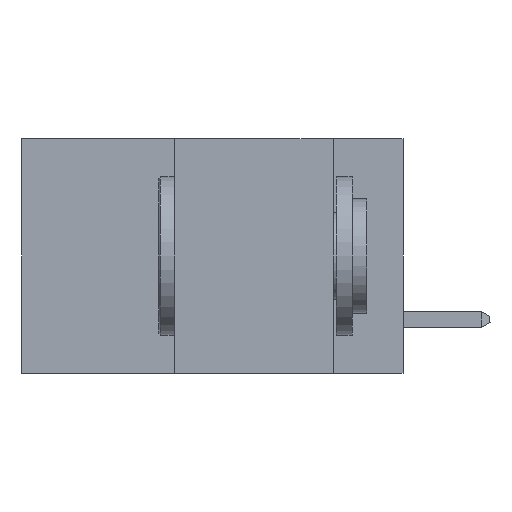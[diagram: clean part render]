
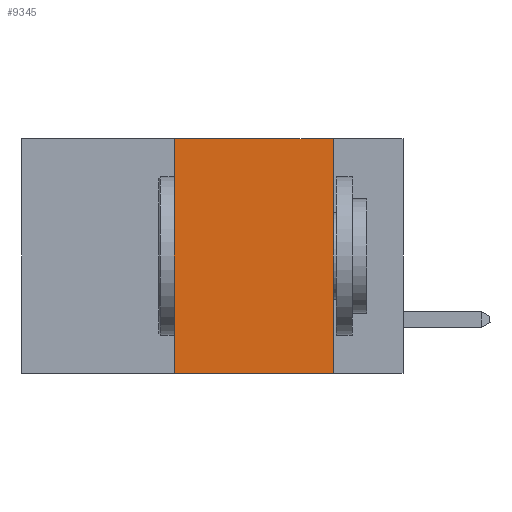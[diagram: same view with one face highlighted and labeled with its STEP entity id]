
A CAD part, left-side view. The second image highlights one B-rep face of the part: STEP entity #9345.
In plain terms, the highlighted planar face has unit normal (-1, 0, 0).
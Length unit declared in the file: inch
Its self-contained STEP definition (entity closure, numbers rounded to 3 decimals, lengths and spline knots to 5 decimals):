
#1799 = CARTESIAN_POINT ( 'NONE',  ( 0., 0.11, -0.37 ) ) ;
#2790 = ORIENTED_EDGE ( 'NONE', *, *, #40341, .F. ) ;
#2924 = ORIENTED_EDGE ( 'NONE', *, *, #37713, .T. ) ;
#2994 = FACE_OUTER_BOUND ( 'NONE', #41935, .T. ) ;
#3256 = LINE ( 'NONE', #39572, #8671 ) ;
#4852 = DIRECTION ( 'NONE',  ( 0., 0., 1. ) ) ;
#5921 = VECTOR ( 'NONE', #29183, 39.37008 ) ;
#8671 = VECTOR ( 'NONE', #4852, 39.37008 ) ;
#9345 = ADVANCED_FACE ( 'NONE', ( #2994 ), #28488, .F. ) ;
#12710 = ORIENTED_EDGE ( 'NONE', *, *, #32119, .F. ) ;
#13232 = VECTOR ( 'NONE', #44209, 39.37008 ) ;
#13265 = CARTESIAN_POINT ( 'NONE',  ( 0., 0.36, -0.37 ) ) ;
#17133 = CARTESIAN_POINT ( 'NONE',  ( 0., 0.6, -0.37 ) ) ;
#17920 = EDGE_CURVE ( 'NONE', #48128, #44416, #3256, .T. ) ;
#19025 = DIRECTION ( 'NONE',  ( 1., 0., 0. ) ) ;
#19349 = CARTESIAN_POINT ( 'NONE',  ( 0., 0.11, 0. ) ) ;
#20032 = AXIS2_PLACEMENT_3D ( 'NONE', #43058, #19025, #24425 ) ;
#23931 = LINE ( 'NONE', #33200, #5921 ) ;
#24425 = DIRECTION ( 'NONE',  ( 0., 0., -1. ) ) ;
#24684 = LINE ( 'NONE', #17133, #13232 ) ;
#26216 = VERTEX_POINT ( 'NONE', #1799 ) ;
#27495 = VECTOR ( 'NONE', #38647, 39.37008 ) ;
#28488 = PLANE ( 'NONE',  #20032 ) ;
#29183 = DIRECTION ( 'NONE',  ( 0., -1., 0. ) ) ;
#29902 = LINE ( 'NONE', #19349, #27495 ) ;
#32119 = EDGE_CURVE ( 'NONE', #44416, #45371, #23931, .T. ) ;
#33200 = CARTESIAN_POINT ( 'NONE',  ( 0., 0.6, 0. ) ) ;
#35949 = CARTESIAN_POINT ( 'NONE',  ( 0., 0.11, 0. ) ) ;
#37713 = EDGE_CURVE ( 'NONE', #48128, #26216, #24684, .T. ) ;
#38647 = DIRECTION ( 'NONE',  ( 0., 0., -1. ) ) ;
#39572 = CARTESIAN_POINT ( 'NONE',  ( 0., 0.36, 0. ) ) ;
#40341 = EDGE_CURVE ( 'NONE', #45371, #26216, #29902, .T. ) ;
#41935 = EDGE_LOOP ( 'NONE', ( #2790, #12710, #49219, #2924 ) ) ;
#43058 = CARTESIAN_POINT ( 'NONE',  ( 0., 0.6, 0. ) ) ;
#44209 = DIRECTION ( 'NONE',  ( 0., -1., 0. ) ) ;
#44416 = VERTEX_POINT ( 'NONE', #48987 ) ;
#45371 = VERTEX_POINT ( 'NONE', #35949 ) ;
#48128 = VERTEX_POINT ( 'NONE', #13265 ) ;
#48987 = CARTESIAN_POINT ( 'NONE',  ( 0., 0.36, 0. ) ) ;
#49219 = ORIENTED_EDGE ( 'NONE', *, *, #17920, .F. ) ;
